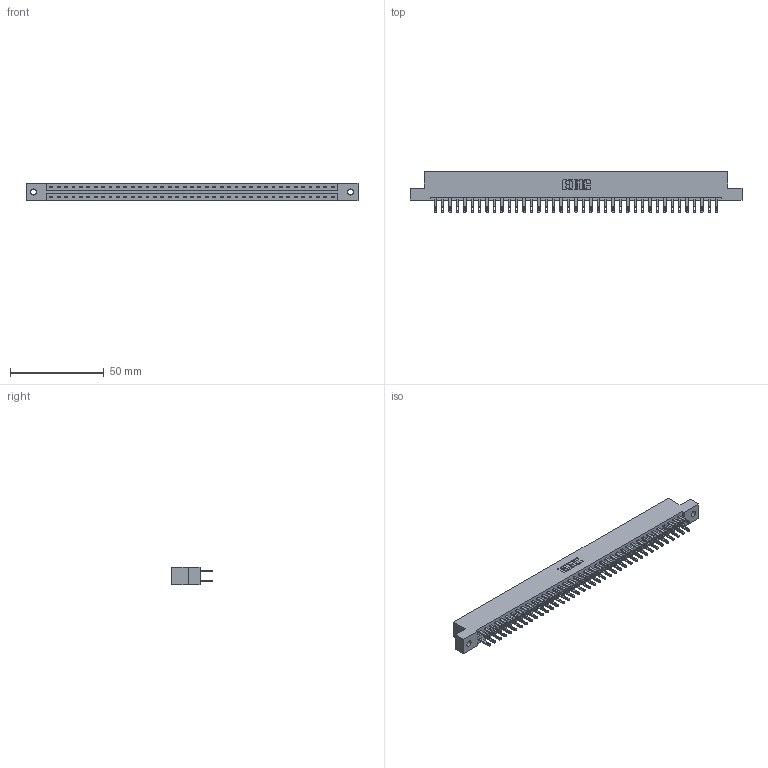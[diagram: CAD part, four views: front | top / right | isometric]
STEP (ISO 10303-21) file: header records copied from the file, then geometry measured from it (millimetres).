
FILE_DESCRIPTION (( 'STEP AP203' ), '1' );
FILE_NAME ('337-078-500-202.STEP', '2019-10-10T11:05:19', ( '' ), ( '' ), 'SwSTEP 2.0', 'SolidWorks 2016', '' );
FILE_SCHEMA (( 'CONFIG_CONTROL_DESIGN' ));
Length unit declared in the file: inch
Products named in the file (3): 345-292-001_345-293-100; 337-078-500-202; 337 Part_Flush Mounting Lugs - 0.128 Dia
Assembly tree (79 placements, depth 2):
  337-078-500-202
    337 Part_Flush Mounting Lugs - 0.128 Dia
    345-292-001_345-293-100  x78
Bounding box: 177.55 x 21.85 x 9.4 mm (x, y, z)
Volume: 18872.9 mm3; surface area: 21899.5 mm2
Topology: 79 solids, 79 shells, 4014 faces, 12245 edges, 8162 vertices
Faces by surface type: plane 2566, cylinder 1448
Entity records: 30559 total; most frequent: CARTESIAN_POINT 5150, ORIENTED_EDGE 5086, DIRECTION 4387, EDGE_CURVE 2543, LINE 2411, VECTOR 2411, VERTEX_POINT 1694, AXIS2_PLACEMENT_3D 988
